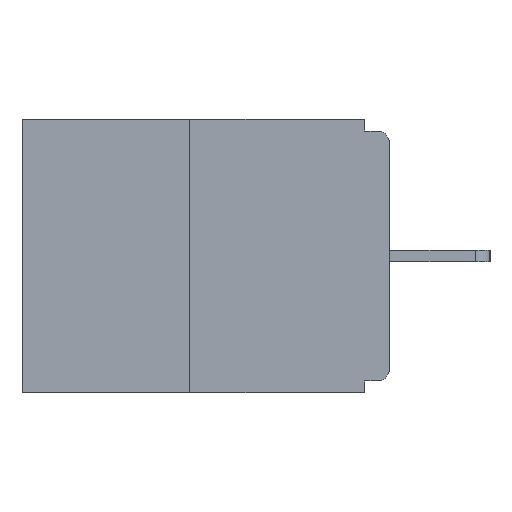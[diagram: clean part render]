
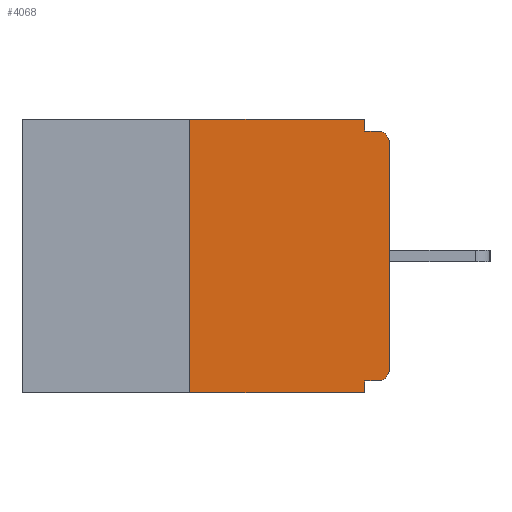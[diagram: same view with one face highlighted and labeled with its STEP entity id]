
A CAD part, left-side view. The second image highlights one B-rep face of the part: STEP entity #4068.
In plain terms, the highlighted planar face has unit normal (-1, 0, 0).
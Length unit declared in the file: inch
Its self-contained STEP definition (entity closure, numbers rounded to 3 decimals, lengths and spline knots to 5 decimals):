
#76 = EDGE_LOOP ( 'NONE', ( #12686, #10558, #3374, #17456, #18708, #11685, #14585, #7205, #16981, #672 ) ) ;
#96 = EDGE_CURVE ( 'NONE', #6838, #12830, #6330, .T. ) ;
#173 = CARTESIAN_POINT ( 'NONE',  ( 0., 0.25, 0. ) ) ;
#284 = VERTEX_POINT ( 'NONE', #14956 ) ;
#359 = CARTESIAN_POINT ( 'NONE',  ( 0., 0.031, -0.015 ) ) ;
#672 = ORIENTED_EDGE ( 'NONE', *, *, #17398, .F. ) ;
#1024 = VECTOR ( 'NONE', #1654, 39.37008 ) ;
#1434 = VERTEX_POINT ( 'NONE', #11183 ) ;
#1654 = DIRECTION ( 'NONE',  ( 0., 0., 1. ) ) ;
#2373 = FACE_OUTER_BOUND ( 'NONE', #76, .T. ) ;
#3374 = ORIENTED_EDGE ( 'NONE', *, *, #16259, .T. ) ;
#3693 = LINE ( 'NONE', #15835, #16845 ) ;
#3792 = CIRCLE ( 'NONE', #16917, 0.015 ) ;
#3805 = DIRECTION ( 'NONE',  ( 0., 0., -1. ) ) ;
#4030 = VECTOR ( 'NONE', #5452, 39.37008 ) ;
#4068 = ADVANCED_FACE ( 'NONE', ( #2373 ), #15744, .F. ) ;
#4616 = CARTESIAN_POINT ( 'NONE',  ( 0., 0.031, -0.343 ) ) ;
#4694 = VECTOR ( 'NONE', #13456, 39.37008 ) ;
#4945 = VERTEX_POINT ( 'NONE', #15855 ) ;
#5105 = DIRECTION ( 'NONE',  ( 0., -1., 0. ) ) ;
#5452 = DIRECTION ( 'NONE',  ( 0., 0., -1. ) ) ;
#5534 = EDGE_CURVE ( 'NONE', #7495, #10905, #18523, .T. ) ;
#6330 = LINE ( 'NONE', #16858, #13098 ) ;
#6530 = DIRECTION ( 'NONE',  ( 0., 0., 1. ) ) ;
#6604 = EDGE_CURVE ( 'NONE', #4945, #12830, #9305, .T. ) ;
#6615 = DIRECTION ( 'NONE',  ( 1., 0., 0. ) ) ;
#6679 = LINE ( 'NONE', #12519, #14977 ) ;
#6838 = VERTEX_POINT ( 'NONE', #359 ) ;
#7205 = ORIENTED_EDGE ( 'NONE', *, *, #6604, .T. ) ;
#7495 = VERTEX_POINT ( 'NONE', #8694 ) ;
#7905 = DIRECTION ( 'NONE',  ( 0., 1., 0. ) ) ;
#8293 = VERTEX_POINT ( 'NONE', #16496 ) ;
#8694 = CARTESIAN_POINT ( 'NONE',  ( 0., 0.25, 0. ) ) ;
#9305 = CIRCLE ( 'NONE', #15058, 0.015 ) ;
#9331 = DIRECTION ( 'NONE',  ( 0., -1., 0. ) ) ;
#9449 = EDGE_CURVE ( 'NONE', #15841, #7495, #14173, .T. ) ;
#10090 = CARTESIAN_POINT ( 'NONE',  ( 0., 0.031, 0. ) ) ;
#10187 = LINE ( 'NONE', #10090, #4030 ) ;
#10558 = ORIENTED_EDGE ( 'NONE', *, *, #9449, .F. ) ;
#10905 = VERTEX_POINT ( 'NONE', #11852 ) ;
#11127 = EDGE_CURVE ( 'NONE', #284, #4945, #11344, .T. ) ;
#11183 = CARTESIAN_POINT ( 'NONE',  ( 0., 0.031, -0.328 ) ) ;
#11344 = LINE ( 'NONE', #14246, #1024 ) ;
#11352 = CARTESIAN_POINT ( 'NONE',  ( 0., 0.46, 0. ) ) ;
#11685 = ORIENTED_EDGE ( 'NONE', *, *, #19778, .T. ) ;
#11811 = VERTEX_POINT ( 'NONE', #4616 ) ;
#11852 = CARTESIAN_POINT ( 'NONE',  ( 0., 0.031, 0. ) ) ;
#11948 = VECTOR ( 'NONE', #6530, 39.37008 ) ;
#12053 = LINE ( 'NONE', #18042, #4694 ) ;
#12519 = CARTESIAN_POINT ( 'NONE',  ( 0., 0., -0.328 ) ) ;
#12686 = ORIENTED_EDGE ( 'NONE', *, *, #5534, .F. ) ;
#12830 = VERTEX_POINT ( 'NONE', #16161 ) ;
#13098 = VECTOR ( 'NONE', #15554, 39.37008 ) ;
#13193 = CARTESIAN_POINT ( 'NONE',  ( 0., 0.015, -0.313 ) ) ;
#13456 = DIRECTION ( 'NONE',  ( 0., 0., -1. ) ) ;
#13752 = AXIS2_PLACEMENT_3D ( 'NONE', #11352, #6615, #17422 ) ;
#14173 = LINE ( 'NONE', #173, #11948 ) ;
#14246 = CARTESIAN_POINT ( 'NONE',  ( 0., 0., 0. ) ) ;
#14480 = EDGE_CURVE ( 'NONE', #1434, #11811, #12053, .T. ) ;
#14585 = ORIENTED_EDGE ( 'NONE', *, *, #11127, .T. ) ;
#14647 = DIRECTION ( 'NONE',  ( -1., 0., 0. ) ) ;
#14956 = CARTESIAN_POINT ( 'NONE',  ( 0., 0., -0.313 ) ) ;
#14977 = VECTOR ( 'NONE', #7905, 39.37008 ) ;
#15058 = AXIS2_PLACEMENT_3D ( 'NONE', #19052, #14647, #3805 ) ;
#15328 = VECTOR ( 'NONE', #9331, 39.37008 ) ;
#15554 = DIRECTION ( 'NONE',  ( 0., -1., 0. ) ) ;
#15744 = PLANE ( 'NONE',  #13752 ) ;
#15835 = CARTESIAN_POINT ( 'NONE',  ( 0., 0.46, -0.343 ) ) ;
#15841 = VERTEX_POINT ( 'NONE', #16792 ) ;
#15855 = CARTESIAN_POINT ( 'NONE',  ( 0., 0., -0.03 ) ) ;
#16075 = DIRECTION ( 'NONE',  ( -1., 0., 0. ) ) ;
#16161 = CARTESIAN_POINT ( 'NONE',  ( 0., 0.015, -0.015 ) ) ;
#16259 = EDGE_CURVE ( 'NONE', #15841, #11811, #3693, .T. ) ;
#16496 = CARTESIAN_POINT ( 'NONE',  ( 0., 0.015, -0.328 ) ) ;
#16792 = CARTESIAN_POINT ( 'NONE',  ( 0., 0.25, -0.343 ) ) ;
#16845 = VECTOR ( 'NONE', #5105, 39.37008 ) ;
#16858 = CARTESIAN_POINT ( 'NONE',  ( 0., 0., -0.015 ) ) ;
#16917 = AXIS2_PLACEMENT_3D ( 'NONE', #13193, #16075, #18910 ) ;
#16981 = ORIENTED_EDGE ( 'NONE', *, *, #96, .F. ) ;
#17398 = EDGE_CURVE ( 'NONE', #10905, #6838, #10187, .T. ) ;
#17422 = DIRECTION ( 'NONE',  ( 0., 0., -1. ) ) ;
#17456 = ORIENTED_EDGE ( 'NONE', *, *, #14480, .F. ) ;
#18042 = CARTESIAN_POINT ( 'NONE',  ( 0., 0.031, -0.343 ) ) ;
#18322 = CARTESIAN_POINT ( 'NONE',  ( 0., 0.46, 0. ) ) ;
#18484 = EDGE_CURVE ( 'NONE', #8293, #1434, #6679, .T. ) ;
#18523 = LINE ( 'NONE', #18322, #15328 ) ;
#18708 = ORIENTED_EDGE ( 'NONE', *, *, #18484, .F. ) ;
#18910 = DIRECTION ( 'NONE',  ( 0., 0., -1. ) ) ;
#19052 = CARTESIAN_POINT ( 'NONE',  ( 0., 0.015, -0.03 ) ) ;
#19778 = EDGE_CURVE ( 'NONE', #8293, #284, #3792, .T. ) ;
